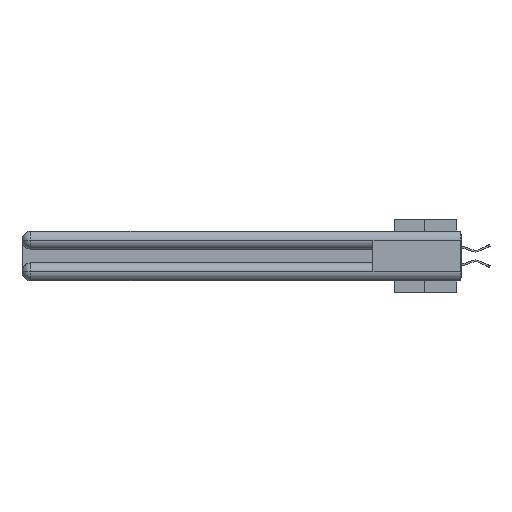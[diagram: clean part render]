
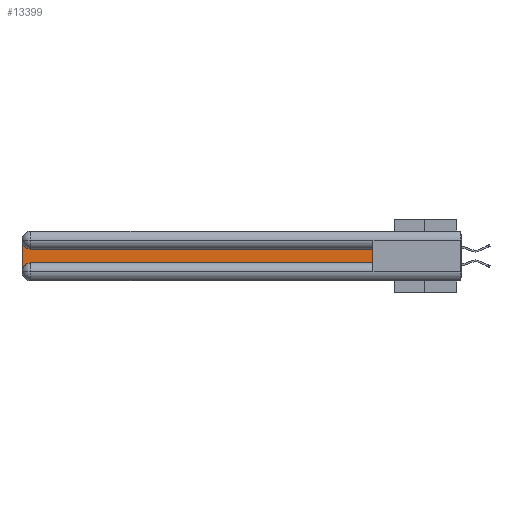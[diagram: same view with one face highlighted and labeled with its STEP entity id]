
A CAD part, left-side view. The second image highlights one B-rep face of the part: STEP entity #13399.
In plain terms, the highlighted planar face has unit normal (-1, 0, 0).
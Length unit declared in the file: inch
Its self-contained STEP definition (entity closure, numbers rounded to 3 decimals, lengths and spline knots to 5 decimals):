
#99 = CARTESIAN_POINT ( 'NONE',  ( 0.075, 0.6, -0.2175 ) ) ;
#545 = LINE ( 'NONE', #16934, #30363 ) ;
#843 = DIRECTION ( 'NONE',  ( 1., 0., 0. ) ) ;
#875 = CARTESIAN_POINT ( 'NONE',  ( 0.075, 0.6, -0.2175 ) ) ;
#1901 = VECTOR ( 'NONE', #13081, 39.37008 ) ;
#2101 = DIRECTION ( 'NONE',  ( 0., 0., -1. ) ) ;
#3395 = PLANE ( 'NONE',  #4318 ) ;
#3941 = VERTEX_POINT ( 'NONE', #19731 ) ;
#4318 = AXIS2_PLACEMENT_3D ( 'NONE', #33670, #843, #19897 ) ;
#4513 = CIRCLE ( 'NONE', #29368, 0.06 ) ;
#6582 = ORIENTED_EDGE ( 'NONE', *, *, #15604, .T. ) ;
#6623 = CARTESIAN_POINT ( 'NONE',  ( 0.075, 3., -0.0625 ) ) ;
#8148 = EDGE_CURVE ( 'NONE', #3941, #28311, #29612, .T. ) ;
#8445 = FACE_OUTER_BOUND ( 'NONE', #23086, .T. ) ;
#10568 = VECTOR ( 'NONE', #16459, 39.37008 ) ;
#11153 = CARTESIAN_POINT ( 'NONE',  ( 0.075, 0.6, -0.2175 ) ) ;
#12433 = ORIENTED_EDGE ( 'NONE', *, *, #18277, .T. ) ;
#12439 = CARTESIAN_POINT ( 'NONE',  ( 0.075, 2.94, -0.0625 ) ) ;
#12553 = DIRECTION ( 'NONE',  ( 1., 0., 0. ) ) ;
#12656 = ORIENTED_EDGE ( 'NONE', *, *, #25332, .T. ) ;
#12808 = VERTEX_POINT ( 'NONE', #27811 ) ;
#12962 = VECTOR ( 'NONE', #21911, 39.37008 ) ;
#13081 = DIRECTION ( 'NONE',  ( 0., 0., -1. ) ) ;
#13307 = CARTESIAN_POINT ( 'NONE',  ( 0.075, 3., -0.2175 ) ) ;
#13342 = CARTESIAN_POINT ( 'NONE',  ( 0.075, 0.6, -0.1225 ) ) ;
#13399 = ADVANCED_FACE ( 'NONE', ( #8445 ), #3395, .F. ) ;
#13929 = EDGE_CURVE ( 'NONE', #12808, #28148, #4513, .T. ) ;
#15604 = EDGE_CURVE ( 'NONE', #28311, #28505, #16151, .T. ) ;
#16151 = LINE ( 'NONE', #99, #10568 ) ;
#16459 = DIRECTION ( 'NONE',  ( 0., -1., 0. ) ) ;
#16934 = CARTESIAN_POINT ( 'NONE',  ( 0.075, 0.6, -0.1225 ) ) ;
#18277 = EDGE_CURVE ( 'NONE', #28505, #27365, #31647, .T. ) ;
#18373 = CARTESIAN_POINT ( 'NONE',  ( 0.075, 2.94, -0.2775 ) ) ;
#18403 = ORIENTED_EDGE ( 'NONE', *, *, #8148, .T. ) ;
#19731 = CARTESIAN_POINT ( 'NONE',  ( 0.075, 3., -0.2775 ) ) ;
#19734 = DIRECTION ( 'NONE',  ( 0., 1., 0. ) ) ;
#19897 = DIRECTION ( 'NONE',  ( 0., 0., -1. ) ) ;
#20326 = AXIS2_PLACEMENT_3D ( 'NONE', #18373, #30017, #2101 ) ;
#21911 = DIRECTION ( 'NONE',  ( 0., 0., 1. ) ) ;
#22039 = ORIENTED_EDGE ( 'NONE', *, *, #13929, .T. ) ;
#23086 = EDGE_LOOP ( 'NONE', ( #12656, #22039, #26616, #18403, #6582, #12433 ) ) ;
#24914 = CARTESIAN_POINT ( 'NONE',  ( 0.075, 2.94, -0.2175 ) ) ;
#25332 = EDGE_CURVE ( 'NONE', #27365, #12808, #545, .T. ) ;
#26616 = ORIENTED_EDGE ( 'NONE', *, *, #33129, .T. ) ;
#27365 = VERTEX_POINT ( 'NONE', #13342 ) ;
#27811 = CARTESIAN_POINT ( 'NONE',  ( 0.075, 2.94, -0.1225 ) ) ;
#27847 = LINE ( 'NONE', #13307, #1901 ) ;
#28148 = VERTEX_POINT ( 'NONE', #6623 ) ;
#28311 = VERTEX_POINT ( 'NONE', #24914 ) ;
#28505 = VERTEX_POINT ( 'NONE', #875 ) ;
#29368 = AXIS2_PLACEMENT_3D ( 'NONE', #12439, #12553, #31973 ) ;
#29612 = CIRCLE ( 'NONE', #20326, 0.06 ) ;
#30017 = DIRECTION ( 'NONE',  ( 1., 0., 0. ) ) ;
#30363 = VECTOR ( 'NONE', #19734, 39.37008 ) ;
#31647 = LINE ( 'NONE', #11153, #12962 ) ;
#31973 = DIRECTION ( 'NONE',  ( 0., 0., -1. ) ) ;
#33129 = EDGE_CURVE ( 'NONE', #28148, #3941, #27847, .T. ) ;
#33670 = CARTESIAN_POINT ( 'NONE',  ( 0.075, 3., -0.1225 ) ) ;
